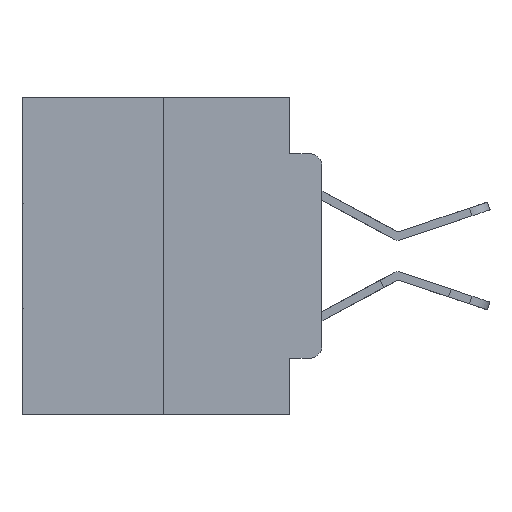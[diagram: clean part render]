
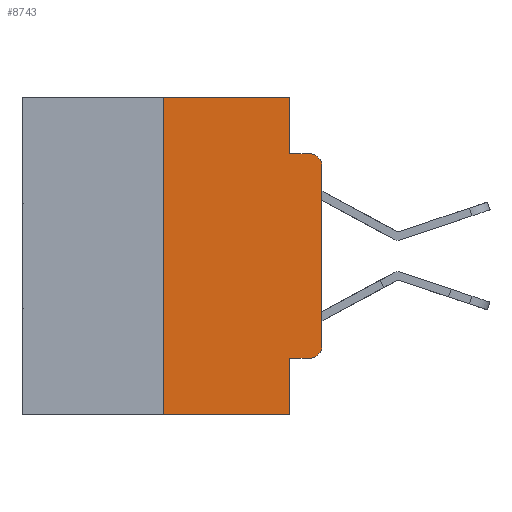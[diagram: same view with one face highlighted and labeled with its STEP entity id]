
A CAD part, left-side view. The second image highlights one B-rep face of the part: STEP entity #8743.
In plain terms, the highlighted planar face has unit normal (-1, 0, 0).
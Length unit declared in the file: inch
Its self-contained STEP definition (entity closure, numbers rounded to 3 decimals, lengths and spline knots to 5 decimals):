
#763 = EDGE_CURVE ( 'NONE', #22803, #8956, #12183, .T. ) ;
#1205 = LINE ( 'NONE', #7126, #12116 ) ;
#1335 = CARTESIAN_POINT ( 'NONE',  ( 0., 0.25, 0. ) ) ;
#1719 = VERTEX_POINT ( 'NONE', #2455 ) ;
#1818 = CARTESIAN_POINT ( 'NONE',  ( 0., 0.02, -0.1085 ) ) ;
#2385 = DIRECTION ( 'NONE',  ( 0., -1., 0. ) ) ;
#2455 = CARTESIAN_POINT ( 'NONE',  ( 0., 0.02, -0.4115 ) ) ;
#2558 = CARTESIAN_POINT ( 'NONE',  ( 0., 0.051, -0.4115 ) ) ;
#2596 = CARTESIAN_POINT ( 'NONE',  ( 0., 0.473, -0.5 ) ) ;
#2963 = CARTESIAN_POINT ( 'NONE',  ( 0., 0.473, 0. ) ) ;
#2973 = VERTEX_POINT ( 'NONE', #19296 ) ;
#3493 = CARTESIAN_POINT ( 'NONE',  ( 0., 0.25, -0.5 ) ) ;
#4042 = DIRECTION ( 'NONE',  ( 0., 0., -1. ) ) ;
#4488 = EDGE_CURVE ( 'NONE', #7491, #24490, #19786, .T. ) ;
#4538 = LINE ( 'NONE', #15487, #10302 ) ;
#4610 = VECTOR ( 'NONE', #4841, 39.37008 ) ;
#4841 = DIRECTION ( 'NONE',  ( 0., -1., 0. ) ) ;
#4892 = VECTOR ( 'NONE', #12419, 39.37008 ) ;
#5083 = PLANE ( 'NONE',  #25201 ) ;
#5148 = VECTOR ( 'NONE', #22118, 39.37008 ) ;
#5377 = ORIENTED_EDGE ( 'NONE', *, *, #6629, .T. ) ;
#5685 = LINE ( 'NONE', #2558, #6357 ) ;
#5982 = CARTESIAN_POINT ( 'NONE',  ( 0., 0.25, 0. ) ) ;
#6357 = VECTOR ( 'NONE', #17857, 39.37008 ) ;
#6397 = VECTOR ( 'NONE', #21477, 39.37008 ) ;
#6613 = CARTESIAN_POINT ( 'NONE',  ( 0., 0.02, -0.0885 ) ) ;
#6629 = EDGE_CURVE ( 'NONE', #13324, #1719, #5685, .T. ) ;
#7044 = ORIENTED_EDGE ( 'NONE', *, *, #4488, .T. ) ;
#7126 = CARTESIAN_POINT ( 'NONE',  ( 0., 0.051, -0.0885 ) ) ;
#7347 = DIRECTION ( 'NONE',  ( 0., 0., -1. ) ) ;
#7491 = VERTEX_POINT ( 'NONE', #27204 ) ;
#7832 = EDGE_CURVE ( 'NONE', #22803, #26970, #22607, .T. ) ;
#8431 = ORIENTED_EDGE ( 'NONE', *, *, #18708, .F. ) ;
#8667 = VECTOR ( 'NONE', #15901, 39.37008 ) ;
#8743 = ADVANCED_FACE ( 'NONE', ( #21226 ), #5083, .F. ) ;
#8956 = VERTEX_POINT ( 'NONE', #1335 ) ;
#9321 = DIRECTION ( 'NONE',  ( 0., -1., 0. ) ) ;
#9348 = CIRCLE ( 'NONE', #10055, 0.02 ) ;
#9784 = ORIENTED_EDGE ( 'NONE', *, *, #7832, .T. ) ;
#10055 = AXIS2_PLACEMENT_3D ( 'NONE', #10087, #25128, #12279 ) ;
#10087 = CARTESIAN_POINT ( 'NONE',  ( 0., 0.02, -0.3915 ) ) ;
#10302 = VECTOR ( 'NONE', #2385, 39.37008 ) ;
#11830 = ORIENTED_EDGE ( 'NONE', *, *, #27310, .T. ) ;
#12001 = EDGE_CURVE ( 'NONE', #13324, #26970, #25145, .T. ) ;
#12116 = VECTOR ( 'NONE', #9321, 39.37008 ) ;
#12183 = LINE ( 'NONE', #5982, #6397 ) ;
#12279 = DIRECTION ( 'NONE',  ( 0., 0., -1. ) ) ;
#12419 = DIRECTION ( 'NONE',  ( 0., 0., -1. ) ) ;
#12901 = CARTESIAN_POINT ( 'NONE',  ( 0., 0., -0.1085 ) ) ;
#13324 = VERTEX_POINT ( 'NONE', #18596 ) ;
#15487 = CARTESIAN_POINT ( 'NONE',  ( 0., 0.473, 0. ) ) ;
#15901 = DIRECTION ( 'NONE',  ( 0., 0., -1. ) ) ;
#16850 = CARTESIAN_POINT ( 'NONE',  ( 0., 0.051, -0.0885 ) ) ;
#17124 = DIRECTION ( 'NONE',  ( -1., 0., 0. ) ) ;
#17857 = DIRECTION ( 'NONE',  ( 0., -1., 0. ) ) ;
#18596 = CARTESIAN_POINT ( 'NONE',  ( 0., 0.051, -0.4115 ) ) ;
#18662 = ORIENTED_EDGE ( 'NONE', *, *, #26621, .T. ) ;
#18708 = EDGE_CURVE ( 'NONE', #2973, #24373, #24166, .T. ) ;
#18921 = CARTESIAN_POINT ( 'NONE',  ( 0., 0.051, 0. ) ) ;
#18953 = EDGE_CURVE ( 'NONE', #8956, #2973, #4538, .T. ) ;
#19296 = CARTESIAN_POINT ( 'NONE',  ( 0., 0.051, 0. ) ) ;
#19786 = LINE ( 'NONE', #24200, #5148 ) ;
#20014 = ORIENTED_EDGE ( 'NONE', *, *, #18953, .F. ) ;
#20407 = DIRECTION ( 'NONE',  ( 1., 0., 0. ) ) ;
#20458 = AXIS2_PLACEMENT_3D ( 'NONE', #1818, #17124, #4042 ) ;
#20706 = ORIENTED_EDGE ( 'NONE', *, *, #763, .F. ) ;
#20912 = CIRCLE ( 'NONE', #20458, 0.02 ) ;
#21185 = VERTEX_POINT ( 'NONE', #6613 ) ;
#21226 = FACE_OUTER_BOUND ( 'NONE', #21660, .T. ) ;
#21477 = DIRECTION ( 'NONE',  ( 0., 0., 1. ) ) ;
#21660 = EDGE_LOOP ( 'NONE', ( #7044, #18662, #24921, #8431, #20014, #20706, #9784, #27547, #5377, #11830 ) ) ;
#22118 = DIRECTION ( 'NONE',  ( 0., 0., 1. ) ) ;
#22607 = LINE ( 'NONE', #2596, #4610 ) ;
#22803 = VERTEX_POINT ( 'NONE', #3493 ) ;
#24166 = LINE ( 'NONE', #18921, #4892 ) ;
#24200 = CARTESIAN_POINT ( 'NONE',  ( 0., 0., 0. ) ) ;
#24373 = VERTEX_POINT ( 'NONE', #16850 ) ;
#24490 = VERTEX_POINT ( 'NONE', #12901 ) ;
#24921 = ORIENTED_EDGE ( 'NONE', *, *, #25237, .F. ) ;
#25128 = DIRECTION ( 'NONE',  ( -1., 0., 0. ) ) ;
#25145 = LINE ( 'NONE', #26545, #8667 ) ;
#25201 = AXIS2_PLACEMENT_3D ( 'NONE', #2963, #20407, #7347 ) ;
#25237 = EDGE_CURVE ( 'NONE', #24373, #21185, #1205, .T. ) ;
#26545 = CARTESIAN_POINT ( 'NONE',  ( 0., 0.051, 0. ) ) ;
#26621 = EDGE_CURVE ( 'NONE', #24490, #21185, #20912, .T. ) ;
#26673 = CARTESIAN_POINT ( 'NONE',  ( 0., 0.051, -0.5 ) ) ;
#26970 = VERTEX_POINT ( 'NONE', #26673 ) ;
#27204 = CARTESIAN_POINT ( 'NONE',  ( 0., 0., -0.3915 ) ) ;
#27310 = EDGE_CURVE ( 'NONE', #1719, #7491, #9348, .T. ) ;
#27547 = ORIENTED_EDGE ( 'NONE', *, *, #12001, .F. ) ;
